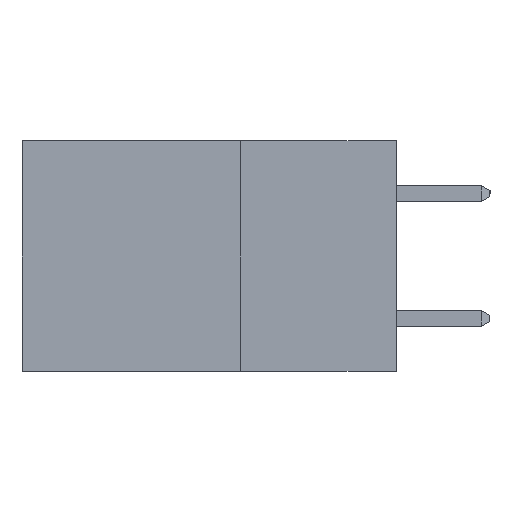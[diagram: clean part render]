
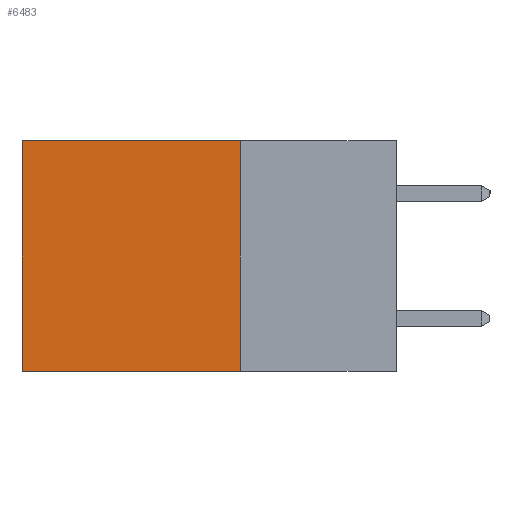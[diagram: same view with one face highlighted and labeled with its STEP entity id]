
A CAD part, left-side view. The second image highlights one B-rep face of the part: STEP entity #6483.
In plain terms, the highlighted planar face has unit normal (-1, 0, 0).
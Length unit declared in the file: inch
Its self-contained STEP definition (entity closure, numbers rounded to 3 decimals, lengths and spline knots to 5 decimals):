
#789 = CARTESIAN_POINT ( 'NONE',  ( 0.2615, 0.25, -0.37 ) ) ;
#1005 = VECTOR ( 'NONE', #9596, 39.37008 ) ;
#1124 = ORIENTED_EDGE ( 'NONE', *, *, #11101, .F. ) ;
#1775 = ORIENTED_EDGE ( 'NONE', *, *, #8607, .F. ) ;
#2157 = CARTESIAN_POINT ( 'NONE',  ( 0.2615, 0.6, -0.37 ) ) ;
#2866 = EDGE_LOOP ( 'NONE', ( #4216, #1775, #1124, #10538 ) ) ;
#4150 = VERTEX_POINT ( 'NONE', #10842 ) ;
#4216 = ORIENTED_EDGE ( 'NONE', *, *, #11537, .T. ) ;
#4452 = LINE ( 'NONE', #10983, #4608 ) ;
#4591 = DIRECTION ( 'NONE',  ( 0., 1., 0. ) ) ;
#4608 = VECTOR ( 'NONE', #4591, 39.37008 ) ;
#5028 = AXIS2_PLACEMENT_3D ( 'NONE', #9489, #8423, #12703 ) ;
#5275 = LINE ( 'NONE', #789, #6381 ) ;
#5307 = CARTESIAN_POINT ( 'NONE',  ( 0.2615, 0.25, -0.37 ) ) ;
#5435 = VERTEX_POINT ( 'NONE', #10560 ) ;
#6090 = LINE ( 'NONE', #10319, #9099 ) ;
#6171 = PLANE ( 'NONE',  #5028 ) ;
#6321 = DIRECTION ( 'NONE',  ( 0., 0., -1. ) ) ;
#6381 = VECTOR ( 'NONE', #6321, 39.37008 ) ;
#6483 = ADVANCED_FACE ( 'NONE', ( #9418 ), #6171, .F. ) ;
#8423 = DIRECTION ( 'NONE',  ( 1., 0., 0. ) ) ;
#8607 = EDGE_CURVE ( 'NONE', #5435, #13740, #13020, .T. ) ;
#9099 = VECTOR ( 'NONE', #9475, 39.37008 ) ;
#9418 = FACE_OUTER_BOUND ( 'NONE', #2866, .T. ) ;
#9475 = DIRECTION ( 'NONE',  ( 0., 0., -1. ) ) ;
#9489 = CARTESIAN_POINT ( 'NONE',  ( 0.2615, 0.25, -0.37 ) ) ;
#9596 = DIRECTION ( 'NONE',  ( 0., 1., 0. ) ) ;
#10319 = CARTESIAN_POINT ( 'NONE',  ( 0.2615, 0.6, -0.37 ) ) ;
#10327 = CARTESIAN_POINT ( 'NONE',  ( 0.2615, 0.25, 0. ) ) ;
#10538 = ORIENTED_EDGE ( 'NONE', *, *, #12413, .T. ) ;
#10560 = CARTESIAN_POINT ( 'NONE',  ( 0.2615, 0.25, -0.37 ) ) ;
#10842 = CARTESIAN_POINT ( 'NONE',  ( 0.2615, 0.6, 0. ) ) ;
#10983 = CARTESIAN_POINT ( 'NONE',  ( 0.2615, 0.25, 0. ) ) ;
#11101 = EDGE_CURVE ( 'NONE', #13061, #5435, #5275, .T. ) ;
#11537 = EDGE_CURVE ( 'NONE', #4150, #13740, #6090, .T. ) ;
#12413 = EDGE_CURVE ( 'NONE', #13061, #4150, #4452, .T. ) ;
#12703 = DIRECTION ( 'NONE',  ( 0., 0., -1. ) ) ;
#13020 = LINE ( 'NONE', #5307, #1005 ) ;
#13061 = VERTEX_POINT ( 'NONE', #10327 ) ;
#13740 = VERTEX_POINT ( 'NONE', #2157 ) ;
